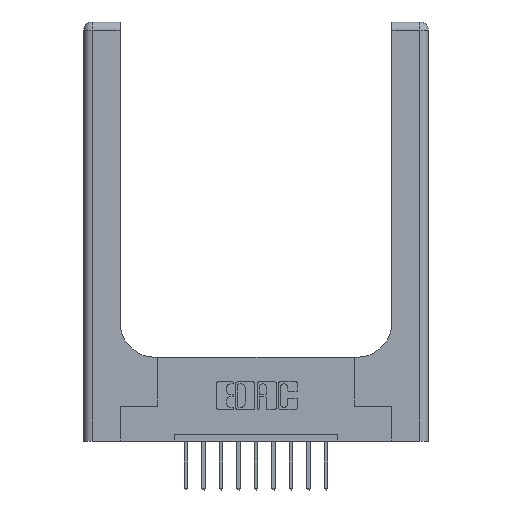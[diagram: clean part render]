
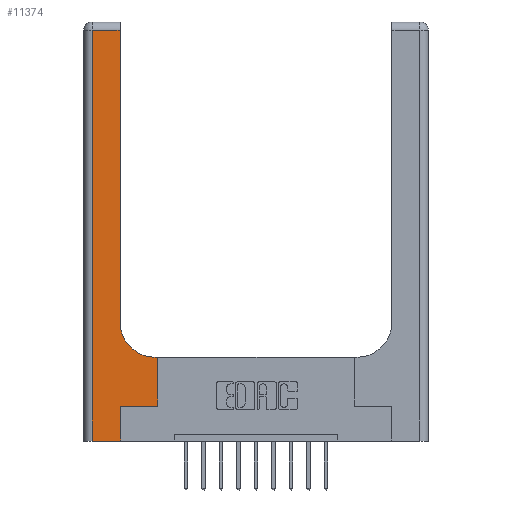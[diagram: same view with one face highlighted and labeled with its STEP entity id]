
A CAD part, top view. The second image highlights one B-rep face of the part: STEP entity #11374.
In plain terms, the highlighted planar face has unit normal (0, 0, 1).
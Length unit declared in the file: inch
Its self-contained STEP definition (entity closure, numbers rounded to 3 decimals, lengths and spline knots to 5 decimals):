
#21 = VECTOR ( 'NONE', #7920, 39.37008 ) ;
#409 = CARTESIAN_POINT ( 'NONE',  ( 0., 0., 0.37 ) ) ;
#1224 = DIRECTION ( 'NONE',  ( -1., 0., 0. ) ) ;
#1242 = AXIS2_PLACEMENT_3D ( 'NONE', #13571, #4962, #1224 ) ;
#1463 = LINE ( 'NONE', #12371, #13603 ) ;
#1473 = EDGE_CURVE ( 'NONE', #9249, #6738, #3845, .T. ) ;
#1821 = DIRECTION ( 'NONE',  ( -1., 0., 0. ) ) ;
#1932 = VERTEX_POINT ( 'NONE', #8365 ) ;
#2077 = CARTESIAN_POINT ( 'NONE',  ( 0.26, 2.94, 0.37 ) ) ;
#2081 = CARTESIAN_POINT ( 'NONE',  ( 0.06, 2.94, 0.37 ) ) ;
#2189 = FACE_OUTER_BOUND ( 'NONE', #6971, .T. ) ;
#2958 = CARTESIAN_POINT ( 'NONE',  ( 0.26, 3., 0.37 ) ) ;
#3201 = VERTEX_POINT ( 'NONE', #2077 ) ;
#3500 = DIRECTION ( 'NONE',  ( 0., 0., -1. ) ) ;
#3845 = LINE ( 'NONE', #409, #4810 ) ;
#4146 = EDGE_CURVE ( 'NONE', #3201, #4240, #12786, .T. ) ;
#4240 = VERTEX_POINT ( 'NONE', #2081 ) ;
#4385 = ORIENTED_EDGE ( 'NONE', *, *, #14538, .T. ) ;
#4810 = VECTOR ( 'NONE', #7500, 39.37008 ) ;
#4962 = DIRECTION ( 'NONE',  ( 0., 0., -1. ) ) ;
#5162 = ORIENTED_EDGE ( 'NONE', *, *, #6495, .T. ) ;
#5257 = VERTEX_POINT ( 'NONE', #12444 ) ;
#6490 = CARTESIAN_POINT ( 'NONE',  ( 0., 2.94, 0.37 ) ) ;
#6495 = EDGE_CURVE ( 'NONE', #4240, #9249, #8617, .T. ) ;
#6588 = CARTESIAN_POINT ( 'NONE',  ( 0.06, 0., 0.37 ) ) ;
#6660 = ORIENTED_EDGE ( 'NONE', *, *, #13636, .T. ) ;
#6738 = VERTEX_POINT ( 'NONE', #9362 ) ;
#6971 = EDGE_LOOP ( 'NONE', ( #4385, #12752, #5162, #14278, #7271, #13153, #12222, #6660, #14867 ) ) ;
#7196 = VECTOR ( 'NONE', #13589, 39.37008 ) ;
#7271 = ORIENTED_EDGE ( 'NONE', *, *, #11509, .T. ) ;
#7375 = CARTESIAN_POINT ( 'NONE',  ( 0.528, 0.6, 0.37 ) ) ;
#7500 = DIRECTION ( 'NONE',  ( 1., 0., 0. ) ) ;
#7895 = VERTEX_POINT ( 'NONE', #9969 ) ;
#7920 = DIRECTION ( 'NONE',  ( 1., 0., 0. ) ) ;
#8365 = CARTESIAN_POINT ( 'NONE',  ( 0.51, 0.6, 0.37 ) ) ;
#8617 = LINE ( 'NONE', #9981, #9164 ) ;
#8828 = AXIS2_PLACEMENT_3D ( 'NONE', #14281, #3500, #14066 ) ;
#9046 = EDGE_CURVE ( 'NONE', #1932, #9054, #14215, .T. ) ;
#9054 = VERTEX_POINT ( 'NONE', #13099 ) ;
#9074 = VERTEX_POINT ( 'NONE', #7375 ) ;
#9164 = VECTOR ( 'NONE', #13388, 39.37008 ) ;
#9240 = VECTOR ( 'NONE', #11250, 39.37008 ) ;
#9249 = VERTEX_POINT ( 'NONE', #6588 ) ;
#9362 = CARTESIAN_POINT ( 'NONE',  ( 0.265, 0., 0.37 ) ) ;
#9427 = LINE ( 'NONE', #2958, #9240 ) ;
#9969 = CARTESIAN_POINT ( 'NONE',  ( 0.265, 0.25, 0.37 ) ) ;
#9981 = CARTESIAN_POINT ( 'NONE',  ( 0.06, 3., 0.37 ) ) ;
#10051 = PLANE ( 'NONE',  #1242 ) ;
#10298 = LINE ( 'NONE', #10779, #7196 ) ;
#10577 = VECTOR ( 'NONE', #1821, 39.37008 ) ;
#10779 = CARTESIAN_POINT ( 'NONE',  ( 0.265, 0., 0.37 ) ) ;
#10915 = EDGE_CURVE ( 'NONE', #5257, #9074, #1463, .T. ) ;
#11250 = DIRECTION ( 'NONE',  ( 0., 1., 0. ) ) ;
#11374 = ADVANCED_FACE ( 'NONE', ( #2189 ), #10051, .F. ) ;
#11509 = EDGE_CURVE ( 'NONE', #6738, #7895, #10298, .T. ) ;
#12222 = ORIENTED_EDGE ( 'NONE', *, *, #10915, .T. ) ;
#12371 = CARTESIAN_POINT ( 'NONE',  ( 0.528, 0.25, 0.37 ) ) ;
#12444 = CARTESIAN_POINT ( 'NONE',  ( 0.528, 0.25, 0.37 ) ) ;
#12470 = DIRECTION ( 'NONE',  ( 0., 1., 0. ) ) ;
#12743 = CARTESIAN_POINT ( 'NONE',  ( 0.265, 0.25, 0.37 ) ) ;
#12752 = ORIENTED_EDGE ( 'NONE', *, *, #4146, .T. ) ;
#12786 = LINE ( 'NONE', #6490, #10577 ) ;
#13099 = CARTESIAN_POINT ( 'NONE',  ( 0.26, 0.85, 0.37 ) ) ;
#13110 = CARTESIAN_POINT ( 'NONE',  ( 0.26, 0.6, 0.37 ) ) ;
#13131 = EDGE_CURVE ( 'NONE', #7895, #5257, #14189, .T. ) ;
#13153 = ORIENTED_EDGE ( 'NONE', *, *, #13131, .T. ) ;
#13388 = DIRECTION ( 'NONE',  ( 0., -1., 0. ) ) ;
#13571 = CARTESIAN_POINT ( 'NONE',  ( 0., 3., 0.37 ) ) ;
#13589 = DIRECTION ( 'NONE',  ( 0., 1., 0. ) ) ;
#13603 = VECTOR ( 'NONE', #12470, 39.37008 ) ;
#13636 = EDGE_CURVE ( 'NONE', #9074, #1932, #14379, .T. ) ;
#14005 = VECTOR ( 'NONE', #14387, 39.37008 ) ;
#14066 = DIRECTION ( 'NONE',  ( 1., 0., 0. ) ) ;
#14189 = LINE ( 'NONE', #12743, #21 ) ;
#14215 = CIRCLE ( 'NONE', #8828, 0.25 ) ;
#14278 = ORIENTED_EDGE ( 'NONE', *, *, #1473, .T. ) ;
#14281 = CARTESIAN_POINT ( 'NONE',  ( 0.51, 0.85, 0.37 ) ) ;
#14379 = LINE ( 'NONE', #13110, #14005 ) ;
#14387 = DIRECTION ( 'NONE',  ( -1., 0., 0. ) ) ;
#14538 = EDGE_CURVE ( 'NONE', #9054, #3201, #9427, .T. ) ;
#14867 = ORIENTED_EDGE ( 'NONE', *, *, #9046, .T. ) ;
